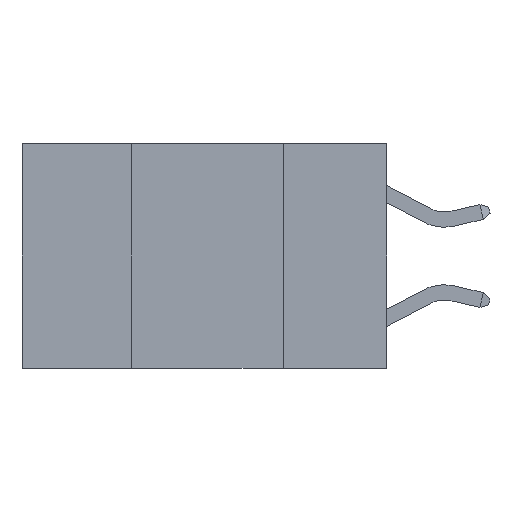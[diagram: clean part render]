
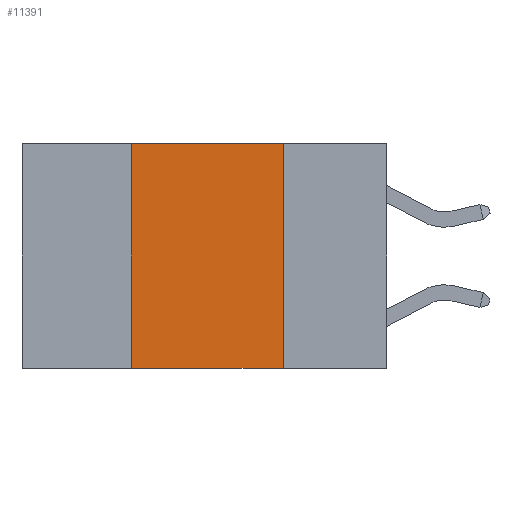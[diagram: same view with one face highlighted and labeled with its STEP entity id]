
A CAD part, left-side view. The second image highlights one B-rep face of the part: STEP entity #11391.
In plain terms, the highlighted planar face has unit normal (-1, 0, 0).
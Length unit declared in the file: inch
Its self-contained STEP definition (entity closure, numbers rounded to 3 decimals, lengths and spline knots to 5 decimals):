
#308 = CARTESIAN_POINT ( 'NONE',  ( 0., 0.17, 0. ) ) ;
#1421 = ORIENTED_EDGE ( 'NONE', *, *, #2009, .F. ) ;
#2009 = EDGE_CURVE ( 'NONE', #10688, #3060, #2208, .T. ) ;
#2208 = LINE ( 'NONE', #308, #11296 ) ;
#2635 = CARTESIAN_POINT ( 'NONE',  ( 0., 0.6, 0. ) ) ;
#3060 = VERTEX_POINT ( 'NONE', #8950 ) ;
#3482 = LINE ( 'NONE', #4298, #12482 ) ;
#3838 = DIRECTION ( 'NONE',  ( 0., 0., -1. ) ) ;
#4247 = EDGE_CURVE ( 'NONE', #10430, #3060, #3482, .T. ) ;
#4292 = EDGE_CURVE ( 'NONE', #5657, #10688, #11777, .T. ) ;
#4298 = CARTESIAN_POINT ( 'NONE',  ( 0., 0.6, -0.37 ) ) ;
#4390 = DIRECTION ( 'NONE',  ( 0., -1., 0. ) ) ;
#5019 = CARTESIAN_POINT ( 'NONE',  ( 0., 0.42, 0. ) ) ;
#5657 = VERTEX_POINT ( 'NONE', #5019 ) ;
#5795 = EDGE_CURVE ( 'NONE', #10430, #5657, #11898, .T. ) ;
#7635 = FACE_OUTER_BOUND ( 'NONE', #12965, .T. ) ;
#7698 = CARTESIAN_POINT ( 'NONE',  ( 0., 0.42, 0. ) ) ;
#8041 = CARTESIAN_POINT ( 'NONE',  ( 0., 0.42, -0.37 ) ) ;
#8698 = VECTOR ( 'NONE', #4390, 39.37008 ) ;
#8950 = CARTESIAN_POINT ( 'NONE',  ( 0., 0.17, -0.37 ) ) ;
#9652 = AXIS2_PLACEMENT_3D ( 'NONE', #2635, #10909, #3838 ) ;
#9734 = PLANE ( 'NONE',  #9652 ) ;
#9981 = DIRECTION ( 'NONE',  ( 0., 0., 1. ) ) ;
#10283 = CARTESIAN_POINT ( 'NONE',  ( 0., 0.6, 0. ) ) ;
#10301 = ORIENTED_EDGE ( 'NONE', *, *, #4247, .T. ) ;
#10430 = VERTEX_POINT ( 'NONE', #8041 ) ;
#10688 = VERTEX_POINT ( 'NONE', #11981 ) ;
#10909 = DIRECTION ( 'NONE',  ( 1., 0., 0. ) ) ;
#11296 = VECTOR ( 'NONE', #13536, 39.37008 ) ;
#11391 = ADVANCED_FACE ( 'NONE', ( #7635 ), #9734, .F. ) ;
#11547 = VECTOR ( 'NONE', #9981, 39.37008 ) ;
#11777 = LINE ( 'NONE', #10283, #8698 ) ;
#11898 = LINE ( 'NONE', #7698, #11547 ) ;
#11981 = CARTESIAN_POINT ( 'NONE',  ( 0., 0.17, 0. ) ) ;
#12108 = ORIENTED_EDGE ( 'NONE', *, *, #5795, .F. ) ;
#12482 = VECTOR ( 'NONE', #14851, 39.37008 ) ;
#12965 = EDGE_LOOP ( 'NONE', ( #1421, #14478, #12108, #10301 ) ) ;
#13536 = DIRECTION ( 'NONE',  ( 0., 0., -1. ) ) ;
#14478 = ORIENTED_EDGE ( 'NONE', *, *, #4292, .F. ) ;
#14851 = DIRECTION ( 'NONE',  ( 0., -1., 0. ) ) ;
